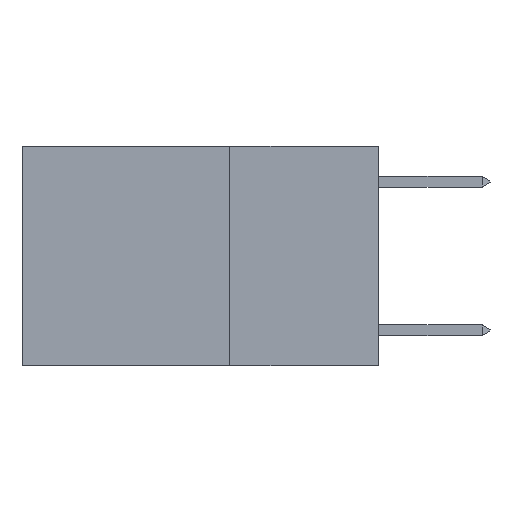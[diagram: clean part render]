
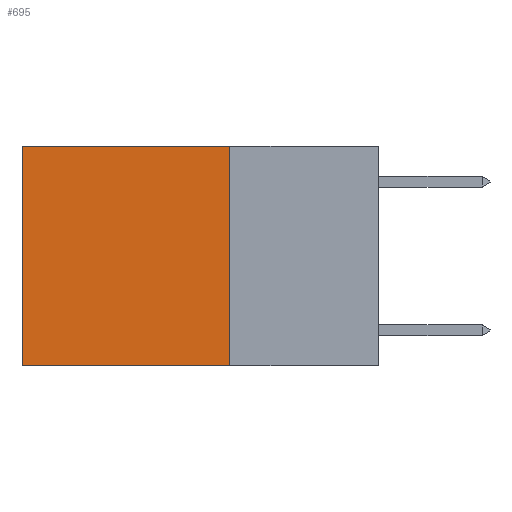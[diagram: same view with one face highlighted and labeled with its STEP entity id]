
A CAD part, left-side view. The second image highlights one B-rep face of the part: STEP entity #695.
In plain terms, the highlighted planar face has unit normal (-1, 0, 0).
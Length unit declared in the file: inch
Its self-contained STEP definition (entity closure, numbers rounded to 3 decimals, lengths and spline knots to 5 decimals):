
#55 = ORIENTED_EDGE ( 'NONE', *, *, #4973, .T. ) ;
#695 = ADVANCED_FACE ( 'NONE', ( #10894 ), #10617, .F. ) ;
#851 = CARTESIAN_POINT ( 'NONE',  ( 0.2625, 0.25, 0. ) ) ;
#1278 = DIRECTION ( 'NONE',  ( 0., 0., -1. ) ) ;
#1573 = LINE ( 'NONE', #5001, #2314 ) ;
#1583 = LINE ( 'NONE', #5014, #5723 ) ;
#1877 = EDGE_CURVE ( 'NONE', #11635, #3144, #9129, .T. ) ;
#2314 = VECTOR ( 'NONE', #9147, 39.37008 ) ;
#2916 = EDGE_LOOP ( 'NONE', ( #55, #3180, #5707, #4951 ) ) ;
#3144 = VERTEX_POINT ( 'NONE', #7881 ) ;
#3180 = ORIENTED_EDGE ( 'NONE', *, *, #11714, .F. ) ;
#3193 = DIRECTION ( 'NONE',  ( 0., 0., -1. ) ) ;
#3839 = AXIS2_PLACEMENT_3D ( 'NONE', #851, #5196, #3193 ) ;
#3937 = LINE ( 'NONE', #8290, #4035 ) ;
#4035 = VECTOR ( 'NONE', #6511, 39.37008 ) ;
#4951 = ORIENTED_EDGE ( 'NONE', *, *, #8586, .T. ) ;
#4973 = EDGE_CURVE ( 'NONE', #13647, #9942, #3937, .T. ) ;
#5001 = CARTESIAN_POINT ( 'NONE',  ( 0.2625, 0.25, -0.37 ) ) ;
#5014 = CARTESIAN_POINT ( 'NONE',  ( 0.2625, 0.25, 0. ) ) ;
#5196 = DIRECTION ( 'NONE',  ( 1., 0., 0. ) ) ;
#5498 = VECTOR ( 'NONE', #1278, 39.37008 ) ;
#5707 = ORIENTED_EDGE ( 'NONE', *, *, #1877, .F. ) ;
#5723 = VECTOR ( 'NONE', #10293, 39.37008 ) ;
#6511 = DIRECTION ( 'NONE',  ( 0., 0., -1. ) ) ;
#7881 = CARTESIAN_POINT ( 'NONE',  ( 0.2625, 0.25, -0.37 ) ) ;
#8290 = CARTESIAN_POINT ( 'NONE',  ( 0.2625, 0.6, 0. ) ) ;
#8586 = EDGE_CURVE ( 'NONE', #11635, #13647, #1583, .T. ) ;
#8871 = CARTESIAN_POINT ( 'NONE',  ( 0.2625, 0.25, 0. ) ) ;
#9129 = LINE ( 'NONE', #11062, #5498 ) ;
#9147 = DIRECTION ( 'NONE',  ( 0., 1., 0. ) ) ;
#9942 = VERTEX_POINT ( 'NONE', #12782 ) ;
#10293 = DIRECTION ( 'NONE',  ( 0., 1., 0. ) ) ;
#10617 = PLANE ( 'NONE',  #3839 ) ;
#10894 = FACE_OUTER_BOUND ( 'NONE', #2916, .T. ) ;
#11062 = CARTESIAN_POINT ( 'NONE',  ( 0.2625, 0.25, 0. ) ) ;
#11635 = VERTEX_POINT ( 'NONE', #8871 ) ;
#11714 = EDGE_CURVE ( 'NONE', #3144, #9942, #1573, .T. ) ;
#12782 = CARTESIAN_POINT ( 'NONE',  ( 0.2625, 0.6, -0.37 ) ) ;
#12969 = CARTESIAN_POINT ( 'NONE',  ( 0.2625, 0.6, 0. ) ) ;
#13647 = VERTEX_POINT ( 'NONE', #12969 ) ;
